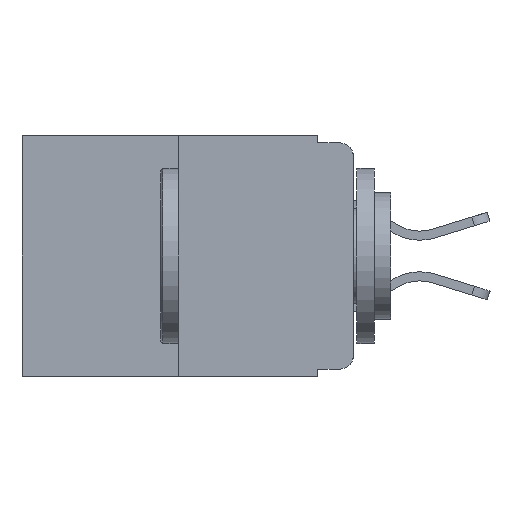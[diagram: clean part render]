
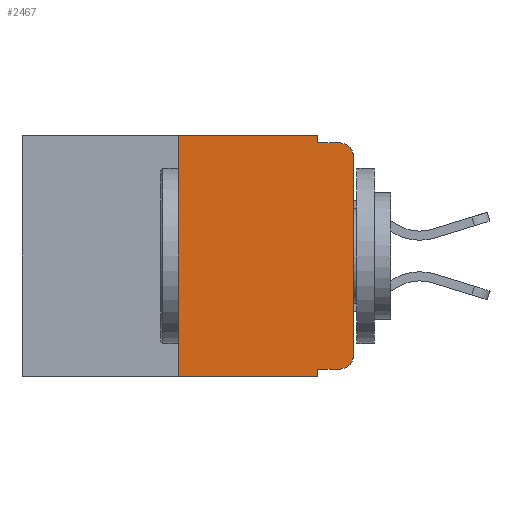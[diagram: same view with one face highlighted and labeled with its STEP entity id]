
A CAD part, left-side view. The second image highlights one B-rep face of the part: STEP entity #2467.
In plain terms, the highlighted planar face has unit normal (-1, 0, 0).
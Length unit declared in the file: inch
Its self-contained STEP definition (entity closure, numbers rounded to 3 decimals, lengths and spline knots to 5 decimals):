
#110 = CARTESIAN_POINT ( 'NONE',  ( 0., 0.02, -0.03 ) ) ;
#164 = CARTESIAN_POINT ( 'NONE',  ( 0., 0.051, 0. ) ) ;
#702 = EDGE_CURVE ( 'NONE', #12829, #8073, #18168, .T. ) ;
#837 = DIRECTION ( 'NONE',  ( 0., 0., 1. ) ) ;
#1998 = ORIENTED_EDGE ( 'NONE', *, *, #21176, .F. ) ;
#2467 = ADVANCED_FACE ( 'NONE', ( #5209 ), #10248, .F. ) ;
#2702 = VERTEX_POINT ( 'NONE', #14444 ) ;
#2974 = CIRCLE ( 'NONE', #13108, 0.02 ) ;
#3285 = DIRECTION ( 'NONE',  ( 0., -1., 0. ) ) ;
#3404 = EDGE_CURVE ( 'NONE', #17708, #12829, #13737, .T. ) ;
#3853 = EDGE_CURVE ( 'NONE', #8426, #18819, #2974, .T. ) ;
#3976 = CARTESIAN_POINT ( 'NONE',  ( 0., 0.02, -0.313 ) ) ;
#4602 = EDGE_CURVE ( 'NONE', #16067, #14788, #6553, .T. ) ;
#4666 = ORIENTED_EDGE ( 'NONE', *, *, #3404, .F. ) ;
#5209 = FACE_OUTER_BOUND ( 'NONE', #9530, .T. ) ;
#5385 = CARTESIAN_POINT ( 'NONE',  ( 0., 0.02, -0.01 ) ) ;
#5615 = ORIENTED_EDGE ( 'NONE', *, *, #18849, .F. ) ;
#5856 = DIRECTION ( 'NONE',  ( 0., 0., -1. ) ) ;
#5932 = VECTOR ( 'NONE', #12058, 39.37008 ) ;
#6097 = ORIENTED_EDGE ( 'NONE', *, *, #20614, .T. ) ;
#6553 = LINE ( 'NONE', #164, #20099 ) ;
#6688 = AXIS2_PLACEMENT_3D ( 'NONE', #110, #18321, #7037 ) ;
#6735 = CARTESIAN_POINT ( 'NONE',  ( 0., 0.051, 0. ) ) ;
#7037 = DIRECTION ( 'NONE',  ( 0., 0., -1. ) ) ;
#7566 = DIRECTION ( 'NONE',  ( 0., 0., -1. ) ) ;
#7668 = VECTOR ( 'NONE', #15797, 39.37008 ) ;
#8073 = VERTEX_POINT ( 'NONE', #5385 ) ;
#8426 = VERTEX_POINT ( 'NONE', #14954 ) ;
#8894 = CARTESIAN_POINT ( 'NONE',  ( 0., 0.25, 0. ) ) ;
#9414 = VERTEX_POINT ( 'NONE', #8894 ) ;
#9530 = EDGE_LOOP ( 'NONE', ( #6097, #11531, #12019, #4666, #1998, #5615, #12875, #18948, #11697, #12804 ) ) ;
#9707 = VECTOR ( 'NONE', #837, 39.37008 ) ;
#9816 = EDGE_CURVE ( 'NONE', #16067, #8426, #10306, .T. ) ;
#9866 = CARTESIAN_POINT ( 'NONE',  ( 0., 0.473, 0. ) ) ;
#10248 = PLANE ( 'NONE',  #20571 ) ;
#10306 = LINE ( 'NONE', #12692, #5932 ) ;
#10454 = DIRECTION ( 'NONE',  ( 0., 0., -1. ) ) ;
#10483 = VECTOR ( 'NONE', #18291, 39.37008 ) ;
#10832 = CARTESIAN_POINT ( 'NONE',  ( 0., 0.25, 0. ) ) ;
#11388 = CARTESIAN_POINT ( 'NONE',  ( 0., 0.25, -0.343 ) ) ;
#11531 = ORIENTED_EDGE ( 'NONE', *, *, #12086, .T. ) ;
#11610 = EDGE_CURVE ( 'NONE', #20109, #14788, #16830, .T. ) ;
#11690 = VECTOR ( 'NONE', #5856, 39.37008 ) ;
#11697 = ORIENTED_EDGE ( 'NONE', *, *, #9816, .T. ) ;
#11912 = DIRECTION ( 'NONE',  ( 0., 0., -1. ) ) ;
#12019 = ORIENTED_EDGE ( 'NONE', *, *, #702, .F. ) ;
#12058 = DIRECTION ( 'NONE',  ( 0., -1., 0. ) ) ;
#12086 = EDGE_CURVE ( 'NONE', #2702, #8073, #16100, .T. ) ;
#12183 = DIRECTION ( 'NONE',  ( -1., 0., 0. ) ) ;
#12437 = LINE ( 'NONE', #20985, #7668 ) ;
#12692 = CARTESIAN_POINT ( 'NONE',  ( 0., 0.051, -0.333 ) ) ;
#12804 = ORIENTED_EDGE ( 'NONE', *, *, #3853, .T. ) ;
#12829 = VERTEX_POINT ( 'NONE', #13113 ) ;
#12875 = ORIENTED_EDGE ( 'NONE', *, *, #11610, .T. ) ;
#13108 = AXIS2_PLACEMENT_3D ( 'NONE', #3976, #12183, #7566 ) ;
#13113 = CARTESIAN_POINT ( 'NONE',  ( 0., 0.051, -0.01 ) ) ;
#13737 = LINE ( 'NONE', #6735, #11690 ) ;
#14418 = LINE ( 'NONE', #10832, #9707 ) ;
#14444 = CARTESIAN_POINT ( 'NONE',  ( 0., 0., -0.03 ) ) ;
#14788 = VERTEX_POINT ( 'NONE', #16587 ) ;
#14954 = CARTESIAN_POINT ( 'NONE',  ( 0., 0.02, -0.333 ) ) ;
#15751 = VECTOR ( 'NONE', #3285, 39.37008 ) ;
#15797 = DIRECTION ( 'NONE',  ( 0., 0., 1. ) ) ;
#16053 = CARTESIAN_POINT ( 'NONE',  ( 0., 0., -0.313 ) ) ;
#16067 = VERTEX_POINT ( 'NONE', #19582 ) ;
#16100 = CIRCLE ( 'NONE', #6688, 0.02 ) ;
#16491 = CARTESIAN_POINT ( 'NONE',  ( 0., 0.051, 0. ) ) ;
#16587 = CARTESIAN_POINT ( 'NONE',  ( 0., 0.051, -0.343 ) ) ;
#16733 = CARTESIAN_POINT ( 'NONE',  ( 0., 0.051, -0.01 ) ) ;
#16818 = CARTESIAN_POINT ( 'NONE',  ( 0., 0.473, 0. ) ) ;
#16830 = LINE ( 'NONE', #18270, #18559 ) ;
#16918 = DIRECTION ( 'NONE',  ( 1., 0., 0. ) ) ;
#17708 = VERTEX_POINT ( 'NONE', #16491 ) ;
#18154 = DIRECTION ( 'NONE',  ( 0., -1., 0. ) ) ;
#18168 = LINE ( 'NONE', #16733, #15751 ) ;
#18181 = LINE ( 'NONE', #9866, #10483 ) ;
#18270 = CARTESIAN_POINT ( 'NONE',  ( 0., 0.473, -0.343 ) ) ;
#18291 = DIRECTION ( 'NONE',  ( 0., -1., 0. ) ) ;
#18321 = DIRECTION ( 'NONE',  ( -1., 0., 0. ) ) ;
#18559 = VECTOR ( 'NONE', #18154, 39.37008 ) ;
#18819 = VERTEX_POINT ( 'NONE', #16053 ) ;
#18849 = EDGE_CURVE ( 'NONE', #20109, #9414, #14418, .T. ) ;
#18948 = ORIENTED_EDGE ( 'NONE', *, *, #4602, .F. ) ;
#19582 = CARTESIAN_POINT ( 'NONE',  ( 0., 0.051, -0.333 ) ) ;
#20099 = VECTOR ( 'NONE', #11912, 39.37008 ) ;
#20109 = VERTEX_POINT ( 'NONE', #11388 ) ;
#20571 = AXIS2_PLACEMENT_3D ( 'NONE', #16818, #16918, #10454 ) ;
#20614 = EDGE_CURVE ( 'NONE', #18819, #2702, #12437, .T. ) ;
#20985 = CARTESIAN_POINT ( 'NONE',  ( 0., 0., 0. ) ) ;
#21176 = EDGE_CURVE ( 'NONE', #9414, #17708, #18181, .T. ) ;
